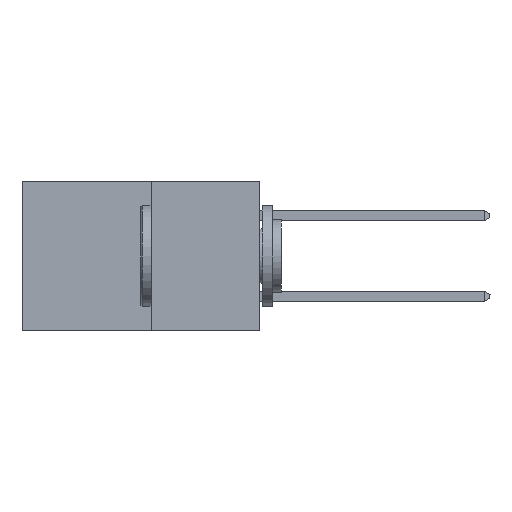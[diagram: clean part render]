
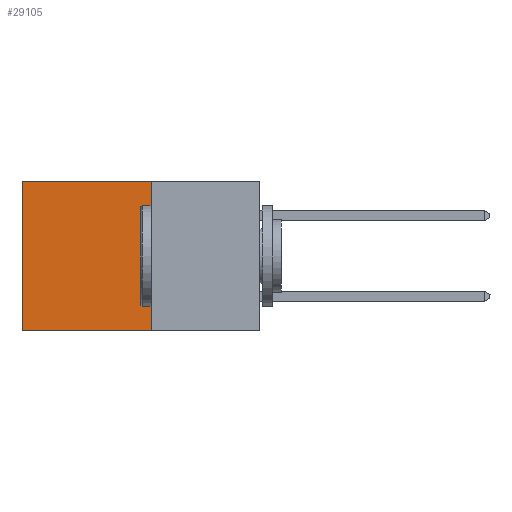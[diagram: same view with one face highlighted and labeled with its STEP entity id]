
A CAD part, left-side view. The second image highlights one B-rep face of the part: STEP entity #29105.
In plain terms, the highlighted planar face has unit normal (-1, 0, 0).
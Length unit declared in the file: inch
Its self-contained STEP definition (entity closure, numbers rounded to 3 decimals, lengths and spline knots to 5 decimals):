
#576 = EDGE_CURVE ( 'NONE', #30857, #17677, #15215, .T. ) ;
#1435 = ORIENTED_EDGE ( 'NONE', *, *, #26871, .T. ) ;
#1526 = EDGE_CURVE ( 'NONE', #12523, #13488, #30953, .T. ) ;
#2782 = ORIENTED_EDGE ( 'NONE', *, *, #4059, .F. ) ;
#2839 = ORIENTED_EDGE ( 'NONE', *, *, #1526, .T. ) ;
#3742 = DIRECTION ( 'NONE',  ( 0., 0., -1. ) ) ;
#4059 = EDGE_CURVE ( 'NONE', #17677, #13488, #18078, .T. ) ;
#4763 = VECTOR ( 'NONE', #17966, 39.37008 ) ;
#6376 = DIRECTION ( 'NONE',  ( 0., 1., 0. ) ) ;
#6391 = CARTESIAN_POINT ( 'NONE',  ( 0.277, 0.27, 0. ) ) ;
#6810 = CARTESIAN_POINT ( 'NONE',  ( 0.277, 0.59, -0.37 ) ) ;
#7268 = DIRECTION ( 'NONE',  ( 1., 0., 0. ) ) ;
#7371 = CARTESIAN_POINT ( 'NONE',  ( 0.277, 0.27, -0.37 ) ) ;
#9814 = EDGE_LOOP ( 'NONE', ( #2839, #2782, #26183, #1435 ) ) ;
#9905 = PLANE ( 'NONE',  #28908 ) ;
#10566 = LINE ( 'NONE', #21297, #23718 ) ;
#12012 = VECTOR ( 'NONE', #3742, 39.37008 ) ;
#12523 = VERTEX_POINT ( 'NONE', #26200 ) ;
#13488 = VERTEX_POINT ( 'NONE', #6810 ) ;
#15215 = LINE ( 'NONE', #30287, #26801 ) ;
#16752 = CARTESIAN_POINT ( 'NONE',  ( 0.277, 0.27, -0.37 ) ) ;
#17677 = VERTEX_POINT ( 'NONE', #23772 ) ;
#17966 = DIRECTION ( 'NONE',  ( 0., 1., 0. ) ) ;
#18078 = LINE ( 'NONE', #16752, #4763 ) ;
#21297 = CARTESIAN_POINT ( 'NONE',  ( 0.277, 0.27, 0. ) ) ;
#23718 = VECTOR ( 'NONE', #6376, 39.37008 ) ;
#23772 = CARTESIAN_POINT ( 'NONE',  ( 0.277, 0.27, -0.37 ) ) ;
#26040 = FACE_OUTER_BOUND ( 'NONE', #9814, .T. ) ;
#26183 = ORIENTED_EDGE ( 'NONE', *, *, #576, .F. ) ;
#26200 = CARTESIAN_POINT ( 'NONE',  ( 0.277, 0.59, 0. ) ) ;
#26801 = VECTOR ( 'NONE', #28479, 39.37008 ) ;
#26871 = EDGE_CURVE ( 'NONE', #30857, #12523, #10566, .T. ) ;
#27254 = DIRECTION ( 'NONE',  ( 0., 0., -1. ) ) ;
#27740 = CARTESIAN_POINT ( 'NONE',  ( 0.277, 0.59, -0.37 ) ) ;
#28479 = DIRECTION ( 'NONE',  ( 0., 0., -1. ) ) ;
#28908 = AXIS2_PLACEMENT_3D ( 'NONE', #7371, #7268, #27254 ) ;
#29105 = ADVANCED_FACE ( 'NONE', ( #26040 ), #9905, .F. ) ;
#30287 = CARTESIAN_POINT ( 'NONE',  ( 0.277, 0.27, -0.37 ) ) ;
#30857 = VERTEX_POINT ( 'NONE', #6391 ) ;
#30953 = LINE ( 'NONE', #27740, #12012 ) ;
